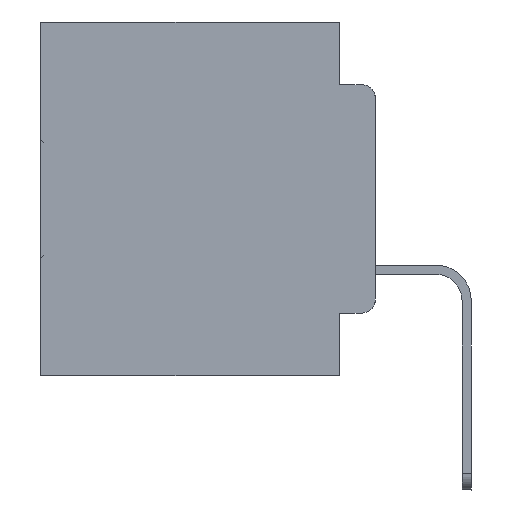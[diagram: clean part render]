
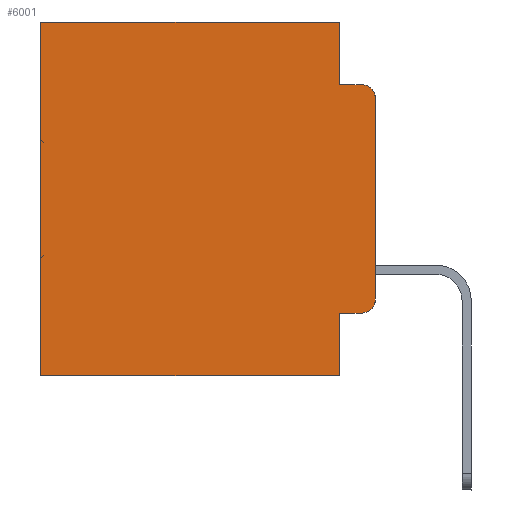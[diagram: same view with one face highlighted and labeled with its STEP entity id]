
A CAD part, left-side view. The second image highlights one B-rep face of the part: STEP entity #6001.
In plain terms, the highlighted planar face has unit normal (-1, 0, 0).
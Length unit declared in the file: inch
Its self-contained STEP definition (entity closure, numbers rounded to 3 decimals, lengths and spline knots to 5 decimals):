
#214 = VERTEX_POINT ( 'NONE', #4848 ) ;
#932 = VERTEX_POINT ( 'NONE', #25198 ) ;
#950 = VERTEX_POINT ( 'NONE', #24766 ) ;
#2000 = DIRECTION ( 'NONE',  ( -1., 0., 0. ) ) ;
#2189 = ORIENTED_EDGE ( 'NONE', *, *, #16780, .F. ) ;
#2753 = LINE ( 'NONE', #21299, #3541 ) ;
#3141 = CARTESIAN_POINT ( 'NONE',  ( 0.298, 0.02, -0.0885 ) ) ;
#3156 = VERTEX_POINT ( 'NONE', #25775 ) ;
#3541 = VECTOR ( 'NONE', #21406, 39.37008 ) ;
#3606 = LINE ( 'NONE', #8601, #22159 ) ;
#4191 = CIRCLE ( 'NONE', #6154, 0.02 ) ;
#4739 = VERTEX_POINT ( 'NONE', #19555 ) ;
#4848 = CARTESIAN_POINT ( 'NONE',  ( 0.298, 0.051, -0.5 ) ) ;
#5192 = CARTESIAN_POINT ( 'NONE',  ( 0.298, 0., 0. ) ) ;
#6001 = ADVANCED_FACE ( 'NONE', ( #6970 ), #23228, .F. ) ;
#6154 = AXIS2_PLACEMENT_3D ( 'NONE', #7090, #7201, #9193 ) ;
#6177 = DIRECTION ( 'NONE',  ( 0., 0., -1. ) ) ;
#6257 = CARTESIAN_POINT ( 'NONE',  ( 0.298, 0.051, 0. ) ) ;
#6282 = VERTEX_POINT ( 'NONE', #6959 ) ;
#6763 = DIRECTION ( 'NONE',  ( 0., 0., -1. ) ) ;
#6959 = CARTESIAN_POINT ( 'NONE',  ( 0.298, 0.02, -0.4115 ) ) ;
#6970 = FACE_OUTER_BOUND ( 'NONE', #25503, .T. ) ;
#6994 = DIRECTION ( 'NONE',  ( 0., 0., -1. ) ) ;
#7090 = CARTESIAN_POINT ( 'NONE',  ( 0.298, 0.02, -0.3915 ) ) ;
#7160 = LINE ( 'NONE', #28159, #21877 ) ;
#7201 = DIRECTION ( 'NONE',  ( -1., 0., 0. ) ) ;
#8338 = LINE ( 'NONE', #30960, #12966 ) ;
#8601 = CARTESIAN_POINT ( 'NONE',  ( 0.298, 0.051, 0. ) ) ;
#8684 = EDGE_CURVE ( 'NONE', #4739, #6282, #20734, .T. ) ;
#8792 = DIRECTION ( 'NONE',  ( 0., 0., -1. ) ) ;
#9193 = DIRECTION ( 'NONE',  ( 0., 0., -1. ) ) ;
#10203 = DIRECTION ( 'NONE',  ( 0., 0., -1. ) ) ;
#10605 = VERTEX_POINT ( 'NONE', #13993 ) ;
#12183 = VECTOR ( 'NONE', #25417, 39.37008 ) ;
#12567 = VERTEX_POINT ( 'NONE', #23463 ) ;
#12966 = VECTOR ( 'NONE', #25865, 39.37008 ) ;
#13324 = LINE ( 'NONE', #5192, #15668 ) ;
#13440 = ORIENTED_EDGE ( 'NONE', *, *, #25594, .F. ) ;
#13613 = DIRECTION ( 'NONE',  ( 0., 1., 0. ) ) ;
#13993 = CARTESIAN_POINT ( 'NONE',  ( 0.298, 0.473, 0. ) ) ;
#15668 = VECTOR ( 'NONE', #10203, 39.37008 ) ;
#16780 = EDGE_CURVE ( 'NONE', #950, #12567, #3606, .T. ) ;
#17435 = EDGE_CURVE ( 'NONE', #950, #10605, #2753, .T. ) ;
#17532 = EDGE_CURVE ( 'NONE', #10605, #21908, #25232, .T. ) ;
#18353 = DIRECTION ( 'NONE',  ( 1., 0., 0. ) ) ;
#19555 = CARTESIAN_POINT ( 'NONE',  ( 0.298, 0.051, -0.4115 ) ) ;
#20516 = DIRECTION ( 'NONE',  ( 0., 0., -1. ) ) ;
#20526 = CARTESIAN_POINT ( 'NONE',  ( 0.298, 0.051, -0.4115 ) ) ;
#20734 = LINE ( 'NONE', #20526, #12183 ) ;
#21299 = CARTESIAN_POINT ( 'NONE',  ( 0.298, 0., 0. ) ) ;
#21406 = DIRECTION ( 'NONE',  ( 0., 1., 0. ) ) ;
#21799 = CARTESIAN_POINT ( 'NONE',  ( 0.298, 0.02, -0.1085 ) ) ;
#21817 = CARTESIAN_POINT ( 'NONE',  ( 0.298, 0.473, 0. ) ) ;
#21877 = VECTOR ( 'NONE', #13613, 39.37008 ) ;
#21908 = VERTEX_POINT ( 'NONE', #21982 ) ;
#21982 = CARTESIAN_POINT ( 'NONE',  ( 0.298, 0.473, -0.5 ) ) ;
#22060 = EDGE_CURVE ( 'NONE', #932, #3156, #13324, .T. ) ;
#22159 = VECTOR ( 'NONE', #6177, 39.37008 ) ;
#22252 = VERTEX_POINT ( 'NONE', #3141 ) ;
#23228 = PLANE ( 'NONE',  #26273 ) ;
#23390 = ORIENTED_EDGE ( 'NONE', *, *, #28532, .T. ) ;
#23463 = CARTESIAN_POINT ( 'NONE',  ( 0.298, 0.051, -0.0885 ) ) ;
#23601 = ORIENTED_EDGE ( 'NONE', *, *, #8684, .T. ) ;
#23655 = EDGE_CURVE ( 'NONE', #6282, #3156, #4191, .T. ) ;
#23682 = VECTOR ( 'NONE', #6994, 39.37008 ) ;
#24649 = EDGE_CURVE ( 'NONE', #4739, #214, #30878, .T. ) ;
#24766 = CARTESIAN_POINT ( 'NONE',  ( 0.298, 0.051, 0. ) ) ;
#25198 = CARTESIAN_POINT ( 'NONE',  ( 0.298, 0., -0.1085 ) ) ;
#25232 = LINE ( 'NONE', #21817, #23682 ) ;
#25417 = DIRECTION ( 'NONE',  ( 0., -1., 0. ) ) ;
#25503 = EDGE_LOOP ( 'NONE', ( #30314, #23390, #13440, #2189, #30423, #26248, #26871, #31658, #23601, #28775 ) ) ;
#25594 = EDGE_CURVE ( 'NONE', #12567, #22252, #8338, .T. ) ;
#25637 = EDGE_CURVE ( 'NONE', #214, #21908, #7160, .T. ) ;
#25775 = CARTESIAN_POINT ( 'NONE',  ( 0.298, 0., -0.3915 ) ) ;
#25865 = DIRECTION ( 'NONE',  ( 0., -1., 0. ) ) ;
#26248 = ORIENTED_EDGE ( 'NONE', *, *, #17532, .T. ) ;
#26273 = AXIS2_PLACEMENT_3D ( 'NONE', #30609, #18353, #20516 ) ;
#26871 = ORIENTED_EDGE ( 'NONE', *, *, #25637, .F. ) ;
#28159 = CARTESIAN_POINT ( 'NONE',  ( 0.298, 0., -0.5 ) ) ;
#28532 = EDGE_CURVE ( 'NONE', #932, #22252, #32164, .T. ) ;
#28775 = ORIENTED_EDGE ( 'NONE', *, *, #23655, .T. ) ;
#29309 = VECTOR ( 'NONE', #8792, 39.37008 ) ;
#30314 = ORIENTED_EDGE ( 'NONE', *, *, #22060, .F. ) ;
#30423 = ORIENTED_EDGE ( 'NONE', *, *, #17435, .T. ) ;
#30609 = CARTESIAN_POINT ( 'NONE',  ( 0.298, 0., 0. ) ) ;
#30878 = LINE ( 'NONE', #6257, #29309 ) ;
#30960 = CARTESIAN_POINT ( 'NONE',  ( 0.298, 0.051, -0.0885 ) ) ;
#31658 = ORIENTED_EDGE ( 'NONE', *, *, #24649, .F. ) ;
#31794 = AXIS2_PLACEMENT_3D ( 'NONE', #21799, #2000, #6763 ) ;
#32164 = CIRCLE ( 'NONE', #31794, 0.02 ) ;
